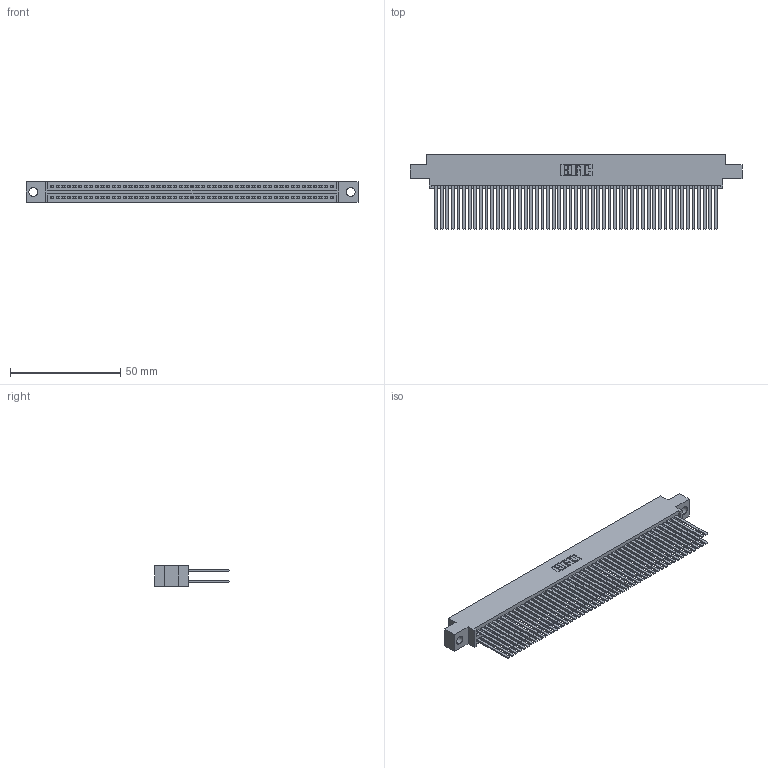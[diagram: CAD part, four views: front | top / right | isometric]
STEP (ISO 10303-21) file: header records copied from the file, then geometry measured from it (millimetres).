
FILE_DESCRIPTION (( 'STEP AP203' ), '1' );
FILE_NAME ('395-102-544-804.STEP', '2018-11-30T08:28:11', ( '' ), ( '' ), 'SwSTEP 2.0', 'SolidWorks 2016', '' );
FILE_SCHEMA (( 'CONFIG_CONTROL_DESIGN' ));
Length unit declared in the file: inch
Products named in the file (3): 345 Part_0.170 Offset - 0.156 Dia-TH; 345-292-001_345-293-144; 395-102-544-804
Assembly tree (103 placements, depth 2):
  395-102-544-804
    345 Part_0.170 Offset - 0.156 Dia-TH
    345-292-001_345-293-144  x102
Bounding box: 150.75 x 33.96 x 9.4 mm (x, y, z)
Volume: 15956.1 mm3; surface area: 27909.5 mm2
Topology: 103 solids, 103 shells, 4618 faces, 13715 edges, 9006 vertices
Faces by surface type: plane 3042, cylinder 1576
Entity records: 38755 total; most frequent: CARTESIAN_POINT 6488, ORIENTED_EDGE 6422, DIRECTION 5707, EDGE_CURVE 3211, VECTOR 2879, LINE 2879, VERTEX_POINT 2138, AXIS2_PLACEMENT_3D 1414
